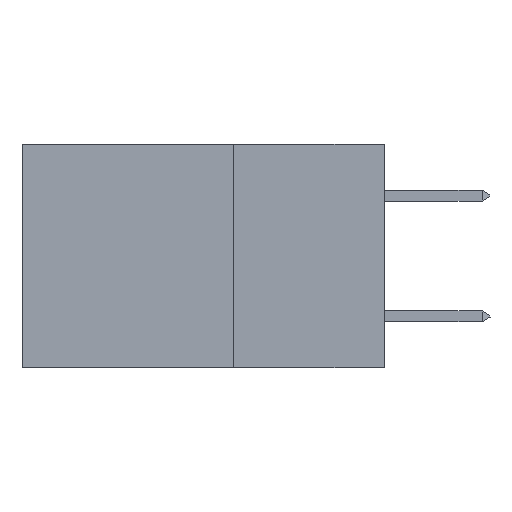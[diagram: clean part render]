
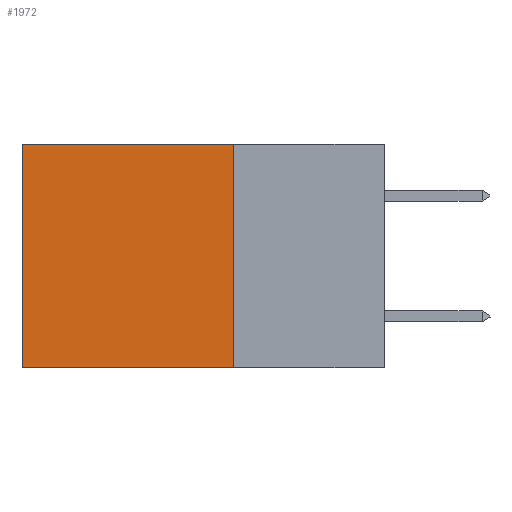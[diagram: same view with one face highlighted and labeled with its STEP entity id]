
A CAD part, left-side view. The second image highlights one B-rep face of the part: STEP entity #1972.
In plain terms, the highlighted planar face has unit normal (-1, 0, 0).
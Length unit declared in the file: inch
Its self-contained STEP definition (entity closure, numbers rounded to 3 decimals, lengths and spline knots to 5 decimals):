
#1972 = ADVANCED_FACE ( 'NONE', ( #6233 ), #13793, .F. ) ;
#2546 = EDGE_CURVE ( 'NONE', #3811, #14627, #4317, .T. ) ;
#3065 = LINE ( 'NONE', #15611, #18793 ) ;
#3431 = CARTESIAN_POINT ( 'NONE',  ( 0.2875, 0.25, 0. ) ) ;
#3811 = VERTEX_POINT ( 'NONE', #15757 ) ;
#4317 = LINE ( 'NONE', #15819, #19697 ) ;
#5537 = LINE ( 'NONE', #22064, #25809 ) ;
#5574 = DIRECTION ( 'NONE',  ( 0., 1., 0. ) ) ;
#5827 = ORIENTED_EDGE ( 'NONE', *, *, #11868, .F. ) ;
#6233 = FACE_OUTER_BOUND ( 'NONE', #12034, .T. ) ;
#7753 = ORIENTED_EDGE ( 'NONE', *, *, #26114, .T. ) ;
#7763 = LINE ( 'NONE', #3431, #8417 ) ;
#8043 = VERTEX_POINT ( 'NONE', #18752 ) ;
#8356 = EDGE_CURVE ( 'NONE', #8043, #13457, #3065, .T. ) ;
#8417 = VECTOR ( 'NONE', #5574, 39.37008 ) ;
#9737 = DIRECTION ( 'NONE',  ( 0., 0., -1. ) ) ;
#10885 = CARTESIAN_POINT ( 'NONE',  ( 0.2875, 0.25, -0.37 ) ) ;
#11868 = EDGE_CURVE ( 'NONE', #13457, #14627, #5537, .T. ) ;
#12034 = EDGE_LOOP ( 'NONE', ( #22581, #5827, #17576, #7753 ) ) ;
#13457 = VERTEX_POINT ( 'NONE', #10885 ) ;
#13709 = DIRECTION ( 'NONE',  ( 0., 0., -1. ) ) ;
#13764 = DIRECTION ( 'NONE',  ( 1., 0., 0. ) ) ;
#13793 = PLANE ( 'NONE',  #25211 ) ;
#14388 = CARTESIAN_POINT ( 'NONE',  ( 0.2875, 0.25, 0. ) ) ;
#14627 = VERTEX_POINT ( 'NONE', #20636 ) ;
#15611 = CARTESIAN_POINT ( 'NONE',  ( 0.2875, 0.25, 0. ) ) ;
#15757 = CARTESIAN_POINT ( 'NONE',  ( 0.2875, 0.6, 0. ) ) ;
#15819 = CARTESIAN_POINT ( 'NONE',  ( 0.2875, 0.6, 0. ) ) ;
#17576 = ORIENTED_EDGE ( 'NONE', *, *, #8356, .F. ) ;
#17644 = DIRECTION ( 'NONE',  ( 0., 0., -1. ) ) ;
#18752 = CARTESIAN_POINT ( 'NONE',  ( 0.2875, 0.25, 0. ) ) ;
#18793 = VECTOR ( 'NONE', #17644, 39.37008 ) ;
#19697 = VECTOR ( 'NONE', #9737, 39.37008 ) ;
#20636 = CARTESIAN_POINT ( 'NONE',  ( 0.2875, 0.6, -0.37 ) ) ;
#22064 = CARTESIAN_POINT ( 'NONE',  ( 0.2875, 0.25, -0.37 ) ) ;
#22581 = ORIENTED_EDGE ( 'NONE', *, *, #2546, .T. ) ;
#24078 = DIRECTION ( 'NONE',  ( 0., 1., 0. ) ) ;
#25211 = AXIS2_PLACEMENT_3D ( 'NONE', #14388, #13764, #13709 ) ;
#25809 = VECTOR ( 'NONE', #24078, 39.37008 ) ;
#26114 = EDGE_CURVE ( 'NONE', #8043, #3811, #7763, .T. ) ;
